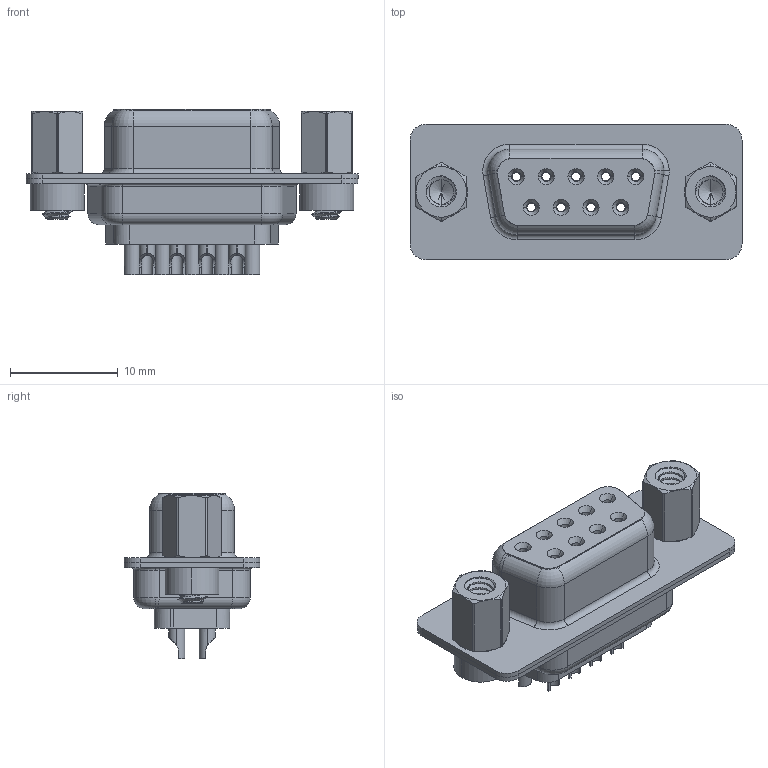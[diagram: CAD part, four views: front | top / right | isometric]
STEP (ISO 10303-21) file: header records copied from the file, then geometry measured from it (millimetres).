
FILE_DESCRIPTION (( 'STEP AP203' ), '1' );
FILE_NAME ('628-009-222-243.STEP', '2020-07-13T18:51:05', ( '' ), ( '' ), 'SwSTEP 2.0', 'SolidWorks 2020', '' );
FILE_SCHEMA (( 'CONFIG_CONTROL_DESIGN' ));
Length unit declared in the file: millimetre
Products named in the file (8): 628 Contact Row 1_22L; 628 Housing_09 LP; 628 4-40 Threaded Rivet; 628 Shell Front_09 Contacts; 628 Contact Row 2_22L; 628-009-222-243; 628 Shell Rear_09 Contacts; 628 4-40 Hex Standoff
Assembly tree (16 placements, depth 2):
  628-009-222-243
    628 Housing_09 LP
    628 Shell Front_09 Contacts
    628 Shell Rear_09 Contacts
    628 Contact Row 1_22L  x5
    628 Contact Row 2_22L  x4
    628 4-40 Threaded Rivet  x2
    628 4-40 Hex Standoff  x2
Bounding box: 30.8 x 12.6 x 15.35 mm (x, y, z)
Volume: 1968.7 mm3; surface area: 4996.8 mm2
Topology: 16 solids, 16 shells, 1202 faces, 3057 edges, 1925 vertices
Faces by surface type: cylinder 432, plane 278, torus 219, bspline 198, cone 75
Entity records: 23768 total; most frequent: CARTESIAN_POINT 9348, ORIENTED_EDGE 2838, DIRECTION 2793, EDGE_CURVE 1419, AXIS2_PLACEMENT_3D 1148, VERTEX_POINT 895, EDGE_LOOP 646, CIRCLE 602
